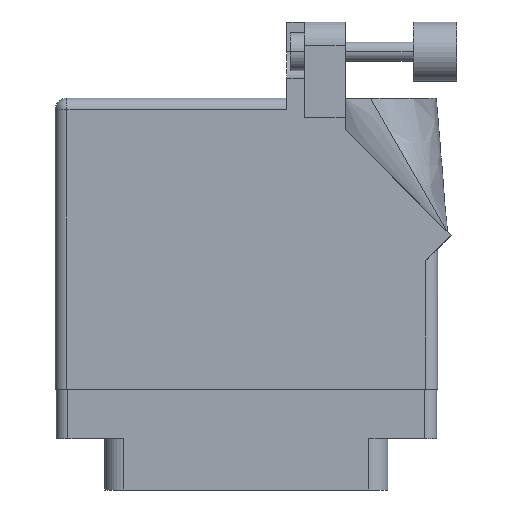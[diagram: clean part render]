
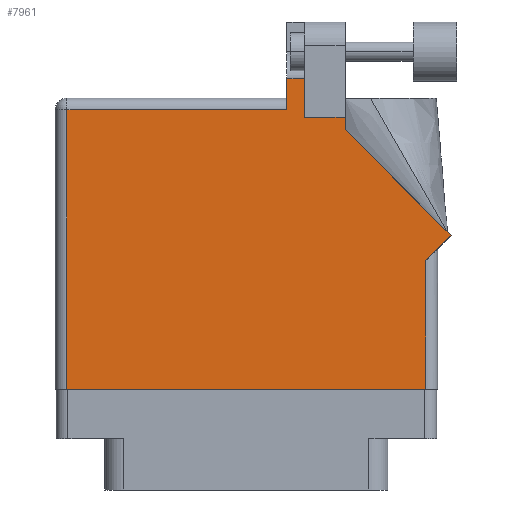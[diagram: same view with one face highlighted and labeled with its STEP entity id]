
A CAD part, front view. The second image highlights one B-rep face of the part: STEP entity #7961.
In plain terms, the highlighted face is planar.
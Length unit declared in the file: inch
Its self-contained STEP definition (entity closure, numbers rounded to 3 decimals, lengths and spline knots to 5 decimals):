
#12 = LINE ( 'NONE', #8048, #32483 ) ;
#117 = VECTOR ( 'NONE', #21586, 39.37008 ) ;
#1690 = CARTESIAN_POINT ( 'NONE',  ( 1.64177, 1.6315, 0. ) ) ;
#1878 = CARTESIAN_POINT ( 'NONE',  ( 0., 1.53, 0. ) ) ;
#1961 = LINE ( 'NONE', #21162, #30195 ) ;
#2107 = DIRECTION ( 'NONE',  ( 0., 0., -1. ) ) ;
#2240 = DIRECTION ( 'NONE',  ( -1., 0., 0. ) ) ;
#2295 = ORIENTED_EDGE ( 'NONE', *, *, #23392, .T. ) ;
#2852 = ORIENTED_EDGE ( 'NONE', *, *, #20706, .T. ) ;
#2978 = CARTESIAN_POINT ( 'NONE',  ( 2.08071, 0.80771, 0. ) ) ;
#3927 = VERTEX_POINT ( 'NONE', #29002 ) ;
#4058 = ORIENTED_EDGE ( 'NONE', *, *, #6833, .T. ) ;
#4594 = EDGE_CURVE ( 'NONE', #16010, #5816, #16623, .T. ) ;
#4694 = VERTEX_POINT ( 'NONE', #8430 ) ;
#4697 = CARTESIAN_POINT ( 'NONE',  ( 2.08071, 0.80771, 0. ) ) ;
#5070 = ORIENTED_EDGE ( 'NONE', *, *, #6113, .T. ) ;
#5319 = ORIENTED_EDGE ( 'NONE', *, *, #21753, .T. ) ;
#5699 = EDGE_CURVE ( 'NONE', #8820, #12213, #33245, .T. ) ;
#5816 = VERTEX_POINT ( 'NONE', #4697 ) ;
#5828 = CARTESIAN_POINT ( 'NONE',  ( 1.524, 1.36442, 0. ) ) ;
#5975 = ORIENTED_EDGE ( 'NONE', *, *, #5699, .T. ) ;
#6015 = EDGE_CURVE ( 'NONE', #20501, #4694, #20594, .T. ) ;
#6113 = EDGE_CURVE ( 'NONE', #12213, #25095, #12, .T. ) ;
#6833 = EDGE_CURVE ( 'NONE', #25095, #14237, #17531, .T. ) ;
#7064 = DIRECTION ( 'NONE',  ( 0., 1., 0. ) ) ;
#7141 = VECTOR ( 'NONE', #29225, 39.37008 ) ;
#7617 = ORIENTED_EDGE ( 'NONE', *, *, #16088, .T. ) ;
#7666 = CARTESIAN_POINT ( 'NONE',  ( 0.062, 1.468, 0. ) ) ;
#7961 = ADVANCED_FACE ( 'NONE', ( #32431 ), #34885, .F. ) ;
#8048 = CARTESIAN_POINT ( 'NONE',  ( 1.217, 1.53, 0. ) ) ;
#8101 = CARTESIAN_POINT ( 'NONE',  ( 1.217, 1.468, 0. ) ) ;
#8424 = VECTOR ( 'NONE', #15369, 39.37008 ) ;
#8430 = CARTESIAN_POINT ( 'NONE',  ( 1.948, 0., 0. ) ) ;
#8820 = VERTEX_POINT ( 'NONE', #26595 ) ;
#9530 = VECTOR ( 'NONE', #31895, 39.37008 ) ;
#10033 = LINE ( 'NONE', #10584, #117 ) ;
#10057 = ORIENTED_EDGE ( 'NONE', *, *, #30539, .T. ) ;
#10371 = DIRECTION ( 'NONE',  ( 0.707, 0.707, 0. ) ) ;
#10584 = CARTESIAN_POINT ( 'NONE',  ( 1.524, 1.36442, 0. ) ) ;
#11577 = VECTOR ( 'NONE', #30359, 39.37008 ) ;
#11639 = LINE ( 'NONE', #29276, #9530 ) ;
#12141 = LINE ( 'NONE', #2978, #28837 ) ;
#12213 = VERTEX_POINT ( 'NONE', #16897 ) ;
#12280 = ORIENTED_EDGE ( 'NONE', *, *, #6015, .T. ) ;
#13277 = CARTESIAN_POINT ( 'NONE',  ( 1.948, 0.675, 0. ) ) ;
#14237 = VERTEX_POINT ( 'NONE', #7666 ) ;
#14748 = VECTOR ( 'NONE', #7064, 39.37008 ) ;
#15369 = DIRECTION ( 'NONE',  ( 0., 1., 0. ) ) ;
#16010 = VERTEX_POINT ( 'NONE', #13277 ) ;
#16088 = EDGE_CURVE ( 'NONE', #5816, #27460, #12141, .T. ) ;
#16282 = EDGE_LOOP ( 'NONE', ( #10057, #5975, #5070, #4058, #2852, #12280, #29330, #31949, #7617, #5319, #2295 ) ) ;
#16623 = LINE ( 'NONE', #26775, #18375 ) ;
#16897 = CARTESIAN_POINT ( 'NONE',  ( 1.217, 1.6315, 0. ) ) ;
#17531 = LINE ( 'NONE', #19003, #26127 ) ;
#18375 = VECTOR ( 'NONE', #10371, 39.37008 ) ;
#18848 = VERTEX_POINT ( 'NONE', #31465 ) ;
#19003 = CARTESIAN_POINT ( 'NONE',  ( 0., 1.468, 0. ) ) ;
#20501 = VERTEX_POINT ( 'NONE', #34198 ) ;
#20539 = CARTESIAN_POINT ( 'NONE',  ( 1.311, 1.43, 0. ) ) ;
#20594 = LINE ( 'NONE', #22115, #11577 ) ;
#20706 = EDGE_CURVE ( 'NONE', #14237, #20501, #1961, .T. ) ;
#21031 = EDGE_CURVE ( 'NONE', #4694, #16010, #30158, .T. ) ;
#21162 = CARTESIAN_POINT ( 'NONE',  ( 0.062, 0., 0. ) ) ;
#21586 = DIRECTION ( 'NONE',  ( 0., 1., 0. ) ) ;
#21753 = EDGE_CURVE ( 'NONE', #27460, #3927, #10033, .T. ) ;
#22115 = CARTESIAN_POINT ( 'NONE',  ( 0., 0., 0. ) ) ;
#22553 = LINE ( 'NONE', #20539, #8424 ) ;
#23392 = EDGE_CURVE ( 'NONE', #3927, #18848, #11639, .T. ) ;
#24703 = DIRECTION ( 'NONE',  ( -1., 0., 0. ) ) ;
#25095 = VERTEX_POINT ( 'NONE', #8101 ) ;
#26127 = VECTOR ( 'NONE', #24703, 39.37008 ) ;
#26595 = CARTESIAN_POINT ( 'NONE',  ( 1.311, 1.6315, 0. ) ) ;
#26775 = CARTESIAN_POINT ( 'NONE',  ( 2.01, 0.737, 0. ) ) ;
#27460 = VERTEX_POINT ( 'NONE', #5828 ) ;
#28837 = VECTOR ( 'NONE', #35505, 39.37008 ) ;
#29002 = CARTESIAN_POINT ( 'NONE',  ( 1.524, 1.43, 0. ) ) ;
#29225 = DIRECTION ( 'NONE',  ( -1., 0., 0. ) ) ;
#29276 = CARTESIAN_POINT ( 'NONE',  ( 1.524, 1.43, 0. ) ) ;
#29330 = ORIENTED_EDGE ( 'NONE', *, *, #21031, .T. ) ;
#30158 = LINE ( 'NONE', #34197, #14748 ) ;
#30195 = VECTOR ( 'NONE', #32051, 39.37008 ) ;
#30359 = DIRECTION ( 'NONE',  ( 1., 0., 0. ) ) ;
#30539 = EDGE_CURVE ( 'NONE', #18848, #8820, #22553, .T. ) ;
#31465 = CARTESIAN_POINT ( 'NONE',  ( 1.311, 1.43, 0. ) ) ;
#31895 = DIRECTION ( 'NONE',  ( -1., 0., 0. ) ) ;
#31949 = ORIENTED_EDGE ( 'NONE', *, *, #4594, .T. ) ;
#32051 = DIRECTION ( 'NONE',  ( 0., -1., 0. ) ) ;
#32431 = FACE_OUTER_BOUND ( 'NONE', #16282, .T. ) ;
#32483 = VECTOR ( 'NONE', #32933, 39.37008 ) ;
#32933 = DIRECTION ( 'NONE',  ( 0., -1., 0. ) ) ;
#33245 = LINE ( 'NONE', #1690, #7141 ) ;
#34197 = CARTESIAN_POINT ( 'NONE',  ( 1.948, 0.737, 0. ) ) ;
#34198 = CARTESIAN_POINT ( 'NONE',  ( 0.062, 0., 0. ) ) ;
#34206 = AXIS2_PLACEMENT_3D ( 'NONE', #1878, #2107, #2240 ) ;
#34885 = PLANE ( 'NONE',  #34206 ) ;
#35505 = DIRECTION ( 'NONE',  ( -0.707, 0.707, 0. ) ) ;
